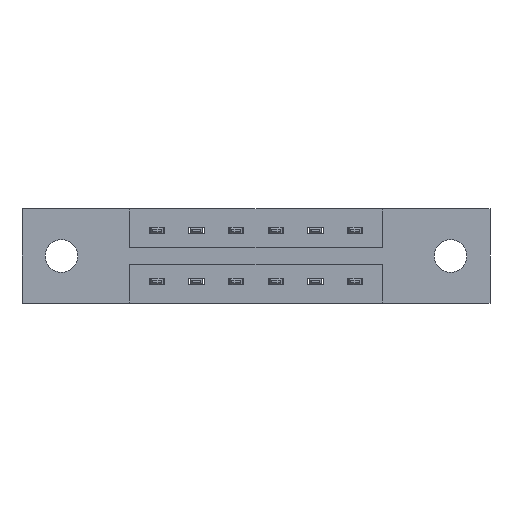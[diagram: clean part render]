
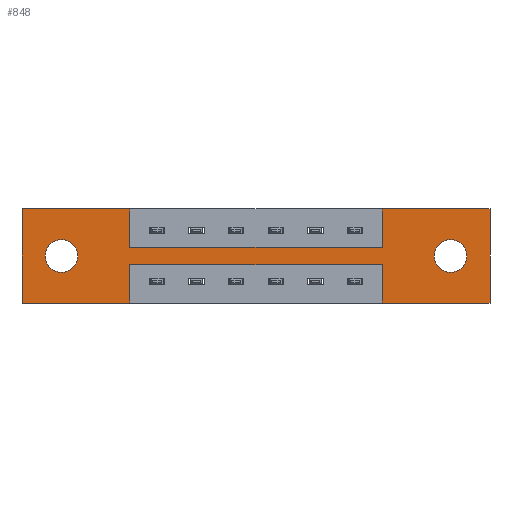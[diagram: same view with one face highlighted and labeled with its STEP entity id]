
A CAD part, front view. The second image highlights one B-rep face of the part: STEP entity #848.
In plain terms, the highlighted planar face has unit normal (0, -1, 0).
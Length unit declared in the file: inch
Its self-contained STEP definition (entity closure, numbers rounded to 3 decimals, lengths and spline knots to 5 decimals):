
#22 = CARTESIAN_POINT ( 'NONE',  ( 1.417, 0., -0.37 ) ) ;
#41 = ORIENTED_EDGE ( 'NONE', *, *, #6911, .T. ) ;
#182 = EDGE_CURVE ( 'NONE', #1986, #4151, #4393, .T. ) ;
#234 = VECTOR ( 'NONE', #2380, 39.37008 ) ;
#601 = VERTEX_POINT ( 'NONE', #4317 ) ;
#848 = ADVANCED_FACE ( 'NONE', ( #6827, #8634, #3151 ), #5512, .T. ) ;
#901 = DIRECTION ( 'NONE',  ( 0., 1., 0. ) ) ;
#963 = CARTESIAN_POINT ( 'NONE',  ( 0., 0., -0.37 ) ) ;
#1022 = DIRECTION ( 'NONE',  ( 0., 0., -1. ) ) ;
#1175 = VECTOR ( 'NONE', #7711, 39.37008 ) ;
#1582 = VERTEX_POINT ( 'NONE', #7027 ) ;
#1587 = CARTESIAN_POINT ( 'NONE',  ( 0.425, 0., -0.15 ) ) ;
#1610 = VECTOR ( 'NONE', #8943, 39.37008 ) ;
#1684 = DIRECTION ( 'NONE',  ( -1., 0., 0. ) ) ;
#1719 = ORIENTED_EDGE ( 'NONE', *, *, #6901, .F. ) ;
#1723 = AXIS2_PLACEMENT_3D ( 'NONE', #4149, #901, #5482 ) ;
#1731 = LINE ( 'NONE', #8720, #3565 ) ;
#1733 = LINE ( 'NONE', #5198, #7225 ) ;
#1738 = DIRECTION ( 'NONE',  ( 0., 0., -1. ) ) ;
#1798 = CARTESIAN_POINT ( 'NONE',  ( 0.425, 0., -0.37 ) ) ;
#1855 = VECTOR ( 'NONE', #1684, 39.37008 ) ;
#1868 = VECTOR ( 'NONE', #6925, 39.37008 ) ;
#1886 = VERTEX_POINT ( 'NONE', #3431 ) ;
#1921 = VERTEX_POINT ( 'NONE', #5136 ) ;
#1956 = VERTEX_POINT ( 'NONE', #4986 ) ;
#1962 = VECTOR ( 'NONE', #4827, 39.37008 ) ;
#1973 = LINE ( 'NONE', #3243, #5808 ) ;
#1986 = VERTEX_POINT ( 'NONE', #8843 ) ;
#2158 = VERTEX_POINT ( 'NONE', #5955 ) ;
#2181 = AXIS2_PLACEMENT_3D ( 'NONE', #2683, #5017, #1738 ) ;
#2380 = DIRECTION ( 'NONE',  ( 1., 0., 0. ) ) ;
#2683 = CARTESIAN_POINT ( 'NONE',  ( 0., 0., -0.37 ) ) ;
#2743 = CARTESIAN_POINT ( 'NONE',  ( 0.425, 0., -0.37 ) ) ;
#2798 = EDGE_CURVE ( 'NONE', #2158, #1921, #1733, .T. ) ;
#2808 = EDGE_LOOP ( 'NONE', ( #7743, #2997 ) ) ;
#2863 = CARTESIAN_POINT ( 'NONE',  ( 0.425, 0., -0.15 ) ) ;
#2997 = ORIENTED_EDGE ( 'NONE', *, *, #7571, .T. ) ;
#3043 = EDGE_CURVE ( 'NONE', #6098, #1582, #1973, .T. ) ;
#3151 = FACE_OUTER_BOUND ( 'NONE', #8294, .T. ) ;
#3231 = CARTESIAN_POINT ( 'NONE',  ( 0., 0., -0.37 ) ) ;
#3236 = VERTEX_POINT ( 'NONE', #6695 ) ;
#3243 = CARTESIAN_POINT ( 'NONE',  ( 0., 0., -0.37 ) ) ;
#3267 = CARTESIAN_POINT ( 'NONE',  ( 1.687, 0., -0.185 ) ) ;
#3431 = CARTESIAN_POINT ( 'NONE',  ( 1.417, 0., 0. ) ) ;
#3556 = DIRECTION ( 'NONE',  ( 1., 0., 0. ) ) ;
#3565 = VECTOR ( 'NONE', #3946, 39.37008 ) ;
#3847 = CARTESIAN_POINT ( 'NONE',  ( 0.155, 0., -0.121 ) ) ;
#3867 = LINE ( 'NONE', #963, #1855 ) ;
#3946 = DIRECTION ( 'NONE',  ( 0., 0., 1. ) ) ;
#3973 = LINE ( 'NONE', #4119, #1962 ) ;
#3976 = DIRECTION ( 'NONE',  ( 0., 0., -1. ) ) ;
#4059 = AXIS2_PLACEMENT_3D ( 'NONE', #3267, #8121, #3976 ) ;
#4091 = EDGE_LOOP ( 'NONE', ( #41, #7254 ) ) ;
#4119 = CARTESIAN_POINT ( 'NONE',  ( 0., 0., 0. ) ) ;
#4149 = CARTESIAN_POINT ( 'NONE',  ( 0.155, 0., -0.185 ) ) ;
#4151 = VERTEX_POINT ( 'NONE', #3847 ) ;
#4208 = LINE ( 'NONE', #1587, #234 ) ;
#4236 = DIRECTION ( 'NONE',  ( 0., 1., 0. ) ) ;
#4276 = VERTEX_POINT ( 'NONE', #1798 ) ;
#4317 = CARTESIAN_POINT ( 'NONE',  ( 1.687, 0., -0.121 ) ) ;
#4362 = LINE ( 'NONE', #5800, #7810 ) ;
#4384 = CARTESIAN_POINT ( 'NONE',  ( 1.687, 0., -0.185 ) ) ;
#4393 = CIRCLE ( 'NONE', #1723, 0.064 ) ;
#4608 = ORIENTED_EDGE ( 'NONE', *, *, #7838, .F. ) ;
#4701 = AXIS2_PLACEMENT_3D ( 'NONE', #4384, #9085, #5089 ) ;
#4710 = ORIENTED_EDGE ( 'NONE', *, *, #6924, .F. ) ;
#4717 = VERTEX_POINT ( 'NONE', #7956 ) ;
#4745 = VECTOR ( 'NONE', #7942, 39.37008 ) ;
#4747 = AXIS2_PLACEMENT_3D ( 'NONE', #8369, #4236, #8977 ) ;
#4751 = LINE ( 'NONE', #6078, #8412 ) ;
#4827 = DIRECTION ( 'NONE',  ( 0., 0., 1. ) ) ;
#4831 = EDGE_CURVE ( 'NONE', #1886, #6458, #4362, .T. ) ;
#4986 = CARTESIAN_POINT ( 'NONE',  ( 0.425, 0., -0.22 ) ) ;
#5017 = DIRECTION ( 'NONE',  ( 0., -1., 0. ) ) ;
#5089 = DIRECTION ( 'NONE',  ( 0., 0., -1. ) ) ;
#5136 = CARTESIAN_POINT ( 'NONE',  ( 0.425, 0., 0. ) ) ;
#5190 = CIRCLE ( 'NONE', #4059, 0.064 ) ;
#5198 = CARTESIAN_POINT ( 'NONE',  ( 0., 0., 0. ) ) ;
#5301 = CIRCLE ( 'NONE', #4747, 0.064 ) ;
#5482 = DIRECTION ( 'NONE',  ( 0., 0., 1. ) ) ;
#5512 = PLANE ( 'NONE',  #2181 ) ;
#5581 = VERTEX_POINT ( 'NONE', #6164 ) ;
#5609 = ORIENTED_EDGE ( 'NONE', *, *, #7746, .F. ) ;
#5718 = LINE ( 'NONE', #8345, #1610 ) ;
#5800 = CARTESIAN_POINT ( 'NONE',  ( 0., 0., 0. ) ) ;
#5808 = VECTOR ( 'NONE', #7279, 39.37008 ) ;
#5843 = ORIENTED_EDGE ( 'NONE', *, *, #7204, .F. ) ;
#5955 = CARTESIAN_POINT ( 'NONE',  ( 0., 0., 0. ) ) ;
#6078 = CARTESIAN_POINT ( 'NONE',  ( 0.425, 0., 0. ) ) ;
#6098 = VERTEX_POINT ( 'NONE', #7771 ) ;
#6164 = CARTESIAN_POINT ( 'NONE',  ( 1.417, 0., -0.22 ) ) ;
#6270 = ORIENTED_EDGE ( 'NONE', *, *, #2798, .F. ) ;
#6389 = ORIENTED_EDGE ( 'NONE', *, *, #8822, .F. ) ;
#6458 = VERTEX_POINT ( 'NONE', #7720 ) ;
#6695 = CARTESIAN_POINT ( 'NONE',  ( 1.687, 0., -0.249 ) ) ;
#6823 = ORIENTED_EDGE ( 'NONE', *, *, #7934, .F. ) ;
#6827 = FACE_BOUND ( 'NONE', #2808, .T. ) ;
#6882 = LINE ( 'NONE', #6961, #1175 ) ;
#6899 = EDGE_CURVE ( 'NONE', #1956, #4276, #7328, .T. ) ;
#6901 = EDGE_CURVE ( 'NONE', #6458, #6098, #5718, .T. ) ;
#6911 = EDGE_CURVE ( 'NONE', #4151, #1986, #5301, .T. ) ;
#6924 = EDGE_CURVE ( 'NONE', #5581, #1956, #6882, .T. ) ;
#6925 = DIRECTION ( 'NONE',  ( 0., 0., -1. ) ) ;
#6961 = CARTESIAN_POINT ( 'NONE',  ( 0.425, 0., -0.22 ) ) ;
#6991 = ORIENTED_EDGE ( 'NONE', *, *, #4831, .F. ) ;
#7027 = CARTESIAN_POINT ( 'NONE',  ( 1.417, 0., -0.37 ) ) ;
#7102 = ORIENTED_EDGE ( 'NONE', *, *, #6899, .F. ) ;
#7204 = EDGE_CURVE ( 'NONE', #4276, #7859, #3867, .T. ) ;
#7225 = VECTOR ( 'NONE', #8183, 39.37008 ) ;
#7254 = ORIENTED_EDGE ( 'NONE', *, *, #182, .T. ) ;
#7279 = DIRECTION ( 'NONE',  ( -1., 0., 0. ) ) ;
#7328 = LINE ( 'NONE', #2743, #1868 ) ;
#7425 = CIRCLE ( 'NONE', #4701, 0.064 ) ;
#7531 = VERTEX_POINT ( 'NONE', #2863 ) ;
#7571 = EDGE_CURVE ( 'NONE', #3236, #601, #7425, .T. ) ;
#7671 = EDGE_CURVE ( 'NONE', #1582, #5581, #8398, .T. ) ;
#7711 = DIRECTION ( 'NONE',  ( -1., 0., 0. ) ) ;
#7720 = CARTESIAN_POINT ( 'NONE',  ( 1.842, 0., 0. ) ) ;
#7743 = ORIENTED_EDGE ( 'NONE', *, *, #7860, .T. ) ;
#7746 = EDGE_CURVE ( 'NONE', #7531, #4717, #4208, .T. ) ;
#7771 = CARTESIAN_POINT ( 'NONE',  ( 1.842, 0., -0.37 ) ) ;
#7810 = VECTOR ( 'NONE', #3556, 39.37008 ) ;
#7838 = EDGE_CURVE ( 'NONE', #4717, #1886, #1731, .T. ) ;
#7859 = VERTEX_POINT ( 'NONE', #3231 ) ;
#7860 = EDGE_CURVE ( 'NONE', #601, #3236, #5190, .T. ) ;
#7934 = EDGE_CURVE ( 'NONE', #1921, #7531, #4751, .T. ) ;
#7942 = DIRECTION ( 'NONE',  ( 0., 0., 1. ) ) ;
#7956 = CARTESIAN_POINT ( 'NONE',  ( 1.417, 0., -0.15 ) ) ;
#8121 = DIRECTION ( 'NONE',  ( 0., 1., 0. ) ) ;
#8183 = DIRECTION ( 'NONE',  ( 1., 0., 0. ) ) ;
#8294 = EDGE_LOOP ( 'NONE', ( #7102, #4710, #8595, #8962, #1719, #6991, #4608, #5609, #6823, #6270, #6389, #5843 ) ) ;
#8345 = CARTESIAN_POINT ( 'NONE',  ( 1.842, 0., 0. ) ) ;
#8369 = CARTESIAN_POINT ( 'NONE',  ( 0.155, 0., -0.185 ) ) ;
#8398 = LINE ( 'NONE', #22, #4745 ) ;
#8412 = VECTOR ( 'NONE', #1022, 39.37008 ) ;
#8595 = ORIENTED_EDGE ( 'NONE', *, *, #7671, .F. ) ;
#8634 = FACE_BOUND ( 'NONE', #4091, .T. ) ;
#8720 = CARTESIAN_POINT ( 'NONE',  ( 1.417, 0., 0. ) ) ;
#8822 = EDGE_CURVE ( 'NONE', #7859, #2158, #3973, .T. ) ;
#8843 = CARTESIAN_POINT ( 'NONE',  ( 0.155, 0., -0.249 ) ) ;
#8943 = DIRECTION ( 'NONE',  ( 0., 0., -1. ) ) ;
#8962 = ORIENTED_EDGE ( 'NONE', *, *, #3043, .F. ) ;
#8977 = DIRECTION ( 'NONE',  ( 0., 0., 1. ) ) ;
#9085 = DIRECTION ( 'NONE',  ( 0., 1., 0. ) ) ;
